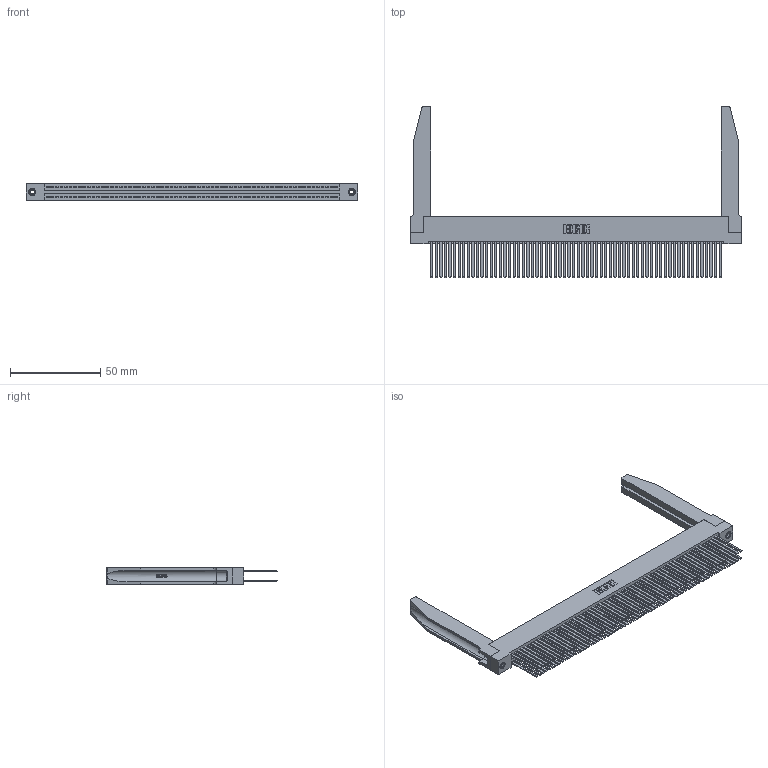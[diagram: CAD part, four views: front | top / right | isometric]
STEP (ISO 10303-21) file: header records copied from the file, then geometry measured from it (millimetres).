
FILE_DESCRIPTION (( 'STEP AP203' ), '1' );
FILE_NAME ('345-128-544-278.STEP', '2019-11-07T09:18:16', ( '' ), ( '' ), 'SwSTEP 2.0', 'SolidWorks 2016', '' );
FILE_SCHEMA (( 'CONFIG_CONTROL_DESIGN' ));
Length unit declared in the file: inch
Products named in the file (5): 345-250-001_345-250-001-102; 345 Part_Flush Mounting Lugs - 0.156 Dia-TH; 345-128-544-278; 345-292-001_345-293-144; 345-220-078_345-220-078
Assembly tree (133 placements, depth 2):
  345-128-544-278
    345 Part_Flush Mounting Lugs - 0.156 Dia-TH
    345-292-001_345-293-144  x128
    345-250-001_345-250-001-102  x2
    345-220-078_345-220-078  x2
Bounding box: 183.79 x 94.92 x 9.4 mm (x, y, z)
Volume: 27622.9 mm3; surface area: 41868.9 mm2
Topology: 133 solids, 133 shells, 5992 faces, 17717 edges, 11630 vertices
Faces by surface type: plane 3934, cylinder 2006, bspline 36, cone 12, torus 4
Entity records: 51810 total; most frequent: CARTESIAN_POINT 9579, ORIENTED_EDGE 8410, DIRECTION 7411, EDGE_CURVE 4205, VECTOR 3727, LINE 3727, VERTEX_POINT 2796, AXIS2_PLACEMENT_3D 1842
